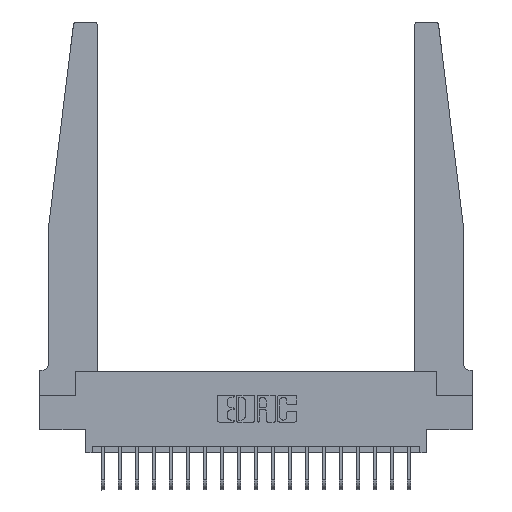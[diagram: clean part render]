
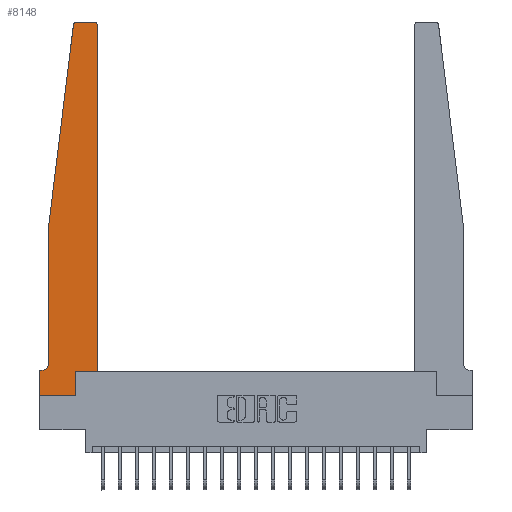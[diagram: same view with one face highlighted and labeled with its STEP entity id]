
A CAD part, top view. The second image highlights one B-rep face of the part: STEP entity #8148.
In plain terms, the highlighted planar face has unit normal (0, 0, 1).
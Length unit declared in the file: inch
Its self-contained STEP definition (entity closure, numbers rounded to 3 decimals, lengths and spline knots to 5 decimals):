
#131 = DIRECTION ( 'NONE',  ( 1., 0., 0. ) ) ;
#240 = ORIENTED_EDGE ( 'NONE', *, *, #18561, .T. ) ;
#547 = VERTEX_POINT ( 'NONE', #3957 ) ;
#739 = CARTESIAN_POINT ( 'NONE',  ( 0.065, 1.25, 0.37 ) ) ;
#777 = ORIENTED_EDGE ( 'NONE', *, *, #1006, .T. ) ;
#1006 = EDGE_CURVE ( 'NONE', #6751, #8554, #10615, .T. ) ;
#1050 = VECTOR ( 'NONE', #16313, 39.37008 ) ;
#1267 = LINE ( 'NONE', #8268, #9822 ) ;
#1278 = ORIENTED_EDGE ( 'NONE', *, *, #19909, .T. ) ;
#1299 = DIRECTION ( 'NONE',  ( 0., 0., 1. ) ) ;
#1387 = VERTEX_POINT ( 'NONE', #2370 ) ;
#1472 = DIRECTION ( 'NONE',  ( -1., 0., 0. ) ) ;
#1500 = CARTESIAN_POINT ( 'NONE',  ( 0.27653, 2.75, 0.37 ) ) ;
#1548 = DIRECTION ( 'NONE',  ( 0., 0., -1. ) ) ;
#1677 = VERTEX_POINT ( 'NONE', #3851 ) ;
#1828 = CARTESIAN_POINT ( 'NONE',  ( 0.395, 2.75, 0.37 ) ) ;
#2012 = VERTEX_POINT ( 'NONE', #1828 ) ;
#2199 = CIRCLE ( 'NONE', #8004, 0.05 ) ;
#2370 = CARTESIAN_POINT ( 'NONE',  ( 0.425, 2.72, 0.37 ) ) ;
#2497 = ORIENTED_EDGE ( 'NONE', *, *, #21036, .T. ) ;
#2549 = ORIENTED_EDGE ( 'NONE', *, *, #19742, .T. ) ;
#2685 = LINE ( 'NONE', #16949, #4824 ) ;
#2948 = LINE ( 'NONE', #4665, #8298 ) ;
#2960 = DIRECTION ( 'NONE',  ( 0., 1., 0. ) ) ;
#3489 = DIRECTION ( 'NONE',  ( 1., 0., 0. ) ) ;
#3638 = EDGE_LOOP ( 'NONE', ( #20546, #20401, #2497, #777, #240, #15055, #12950, #12652, #2549, #16649, #1278, #21168 ) ) ;
#3851 = CARTESIAN_POINT ( 'NONE',  ( 0., 0., 0.37 ) ) ;
#3876 = AXIS2_PLACEMENT_3D ( 'NONE', #17509, #15633, #19239 ) ;
#3901 = CARTESIAN_POINT ( 'NONE',  ( 0., 0.1875, 0.37 ) ) ;
#3957 = CARTESIAN_POINT ( 'NONE',  ( 0.24675, 2.72367, 0.37 ) ) ;
#4323 = CARTESIAN_POINT ( 'NONE',  ( 0., 0., 0.37 ) ) ;
#4665 = CARTESIAN_POINT ( 'NONE',  ( 0.425, 0.18, 0.37 ) ) ;
#4824 = VECTOR ( 'NONE', #8410, 39.37008 ) ;
#4849 = VECTOR ( 'NONE', #6434, 39.37008 ) ;
#5309 = VERTEX_POINT ( 'NONE', #20400 ) ;
#5397 = EDGE_CURVE ( 'NONE', #17538, #5309, #2685, .T. ) ;
#5439 = LINE ( 'NONE', #4323, #15097 ) ;
#5919 = EDGE_CURVE ( 'NONE', #20452, #7006, #21433, .T. ) ;
#6371 = PLANE ( 'NONE',  #19102 ) ;
#6434 = DIRECTION ( 'NONE',  ( 0., -1., 0. ) ) ;
#6709 = LINE ( 'NONE', #11470, #4849 ) ;
#6751 = VERTEX_POINT ( 'NONE', #10150 ) ;
#7006 = VERTEX_POINT ( 'NONE', #7417 ) ;
#7417 = CARTESIAN_POINT ( 'NONE',  ( 0.425, 0.18, 0.37 ) ) ;
#7418 = EDGE_CURVE ( 'NONE', #1387, #2012, #8379, .T. ) ;
#8004 = AXIS2_PLACEMENT_3D ( 'NONE', #13655, #1548, #1472 ) ;
#8144 = EDGE_CURVE ( 'NONE', #17960, #547, #8825, .T. ) ;
#8148 = ADVANCED_FACE ( 'NONE', ( #16048 ), #6371, .T. ) ;
#8268 = CARTESIAN_POINT ( 'NONE',  ( 0.25, 2.75, 0.37 ) ) ;
#8298 = VECTOR ( 'NONE', #2960, 39.37008 ) ;
#8379 = CIRCLE ( 'NONE', #3876, 0.03 ) ;
#8410 = DIRECTION ( 'NONE',  ( -1., 0., 0. ) ) ;
#8554 = VERTEX_POINT ( 'NONE', #14974 ) ;
#8825 = CIRCLE ( 'NONE', #10916, 0.03 ) ;
#8949 = DIRECTION ( 'NONE',  ( 0., 0., 1. ) ) ;
#9344 = DIRECTION ( 'NONE',  ( 0., -1., 0. ) ) ;
#9662 = EDGE_CURVE ( 'NONE', #2012, #17960, #1267, .T. ) ;
#9717 = CARTESIAN_POINT ( 'NONE',  ( 0.065, 1.25, 0.37 ) ) ;
#9822 = VECTOR ( 'NONE', #9900, 39.37008 ) ;
#9900 = DIRECTION ( 'NONE',  ( -1., 0., 0. ) ) ;
#10150 = CARTESIAN_POINT ( 'NONE',  ( 0.065, 1.25, 0.37 ) ) ;
#10340 = CARTESIAN_POINT ( 'NONE',  ( 0.015, 0.1875, 0.37 ) ) ;
#10615 = LINE ( 'NONE', #739, #18126 ) ;
#10916 = AXIS2_PLACEMENT_3D ( 'NONE', #21249, #1299, #131 ) ;
#11157 = DIRECTION ( 'NONE',  ( 1., 0., 0. ) ) ;
#11276 = CARTESIAN_POINT ( 'NONE',  ( 0.2605, 0.18, 0.37 ) ) ;
#11470 = CARTESIAN_POINT ( 'NONE',  ( 0., 0., 0.37 ) ) ;
#11783 = EDGE_CURVE ( 'NONE', #1677, #15023, #5439, .T. ) ;
#12076 = LINE ( 'NONE', #11276, #21714 ) ;
#12652 = ORIENTED_EDGE ( 'NONE', *, *, #11783, .T. ) ;
#12950 = ORIENTED_EDGE ( 'NONE', *, *, #19196, .T. ) ;
#13124 = CARTESIAN_POINT ( 'NONE',  ( 0.2605, 0., 0.37 ) ) ;
#13655 = CARTESIAN_POINT ( 'NONE',  ( 0.015, 0.2375, 0.37 ) ) ;
#14643 = DIRECTION ( 'NONE',  ( 0., 1., 0. ) ) ;
#14668 = LINE ( 'NONE', #9717, #20303 ) ;
#14974 = CARTESIAN_POINT ( 'NONE',  ( 0.065, 0.2375, 0.37 ) ) ;
#15023 = VERTEX_POINT ( 'NONE', #13124 ) ;
#15055 = ORIENTED_EDGE ( 'NONE', *, *, #5397, .T. ) ;
#15097 = VECTOR ( 'NONE', #11157, 39.37008 ) ;
#15633 = DIRECTION ( 'NONE',  ( 0., 0., 1. ) ) ;
#16048 = FACE_OUTER_BOUND ( 'NONE', #3638, .T. ) ;
#16313 = DIRECTION ( 'NONE',  ( 1., 0., 0. ) ) ;
#16649 = ORIENTED_EDGE ( 'NONE', *, *, #5919, .T. ) ;
#16949 = CARTESIAN_POINT ( 'NONE',  ( 0.065, 0.1875, 0.37 ) ) ;
#17509 = CARTESIAN_POINT ( 'NONE',  ( 0.395, 2.72, 0.37 ) ) ;
#17538 = VERTEX_POINT ( 'NONE', #10340 ) ;
#17960 = VERTEX_POINT ( 'NONE', #1500 ) ;
#18126 = VECTOR ( 'NONE', #9344, 39.37008 ) ;
#18561 = EDGE_CURVE ( 'NONE', #8554, #17538, #2199, .T. ) ;
#19102 = AXIS2_PLACEMENT_3D ( 'NONE', #3901, #8949, #3489 ) ;
#19196 = EDGE_CURVE ( 'NONE', #5309, #1677, #6709, .T. ) ;
#19239 = DIRECTION ( 'NONE',  ( 1., 0., 0. ) ) ;
#19742 = EDGE_CURVE ( 'NONE', #15023, #20452, #12076, .T. ) ;
#19909 = EDGE_CURVE ( 'NONE', #7006, #1387, #2948, .T. ) ;
#20303 = VECTOR ( 'NONE', #21720, 39.37008 ) ;
#20313 = CARTESIAN_POINT ( 'NONE',  ( 0.2605, 0.18, 0.37 ) ) ;
#20400 = CARTESIAN_POINT ( 'NONE',  ( 0., 0.1875, 0.37 ) ) ;
#20401 = ORIENTED_EDGE ( 'NONE', *, *, #8144, .T. ) ;
#20411 = CARTESIAN_POINT ( 'NONE',  ( 0.425, 0.18, 0.37 ) ) ;
#20452 = VERTEX_POINT ( 'NONE', #20313 ) ;
#20546 = ORIENTED_EDGE ( 'NONE', *, *, #9662, .T. ) ;
#21036 = EDGE_CURVE ( 'NONE', #547, #6751, #14668, .T. ) ;
#21168 = ORIENTED_EDGE ( 'NONE', *, *, #7418, .T. ) ;
#21249 = CARTESIAN_POINT ( 'NONE',  ( 0.27653, 2.72, 0.37 ) ) ;
#21433 = LINE ( 'NONE', #20411, #1050 ) ;
#21714 = VECTOR ( 'NONE', #14643, 39.37008 ) ;
#21720 = DIRECTION ( 'NONE',  ( -0.122, -0.992, 0. ) ) ;
